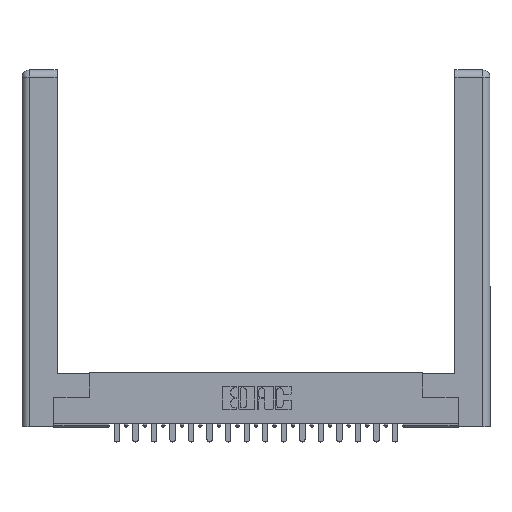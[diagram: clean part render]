
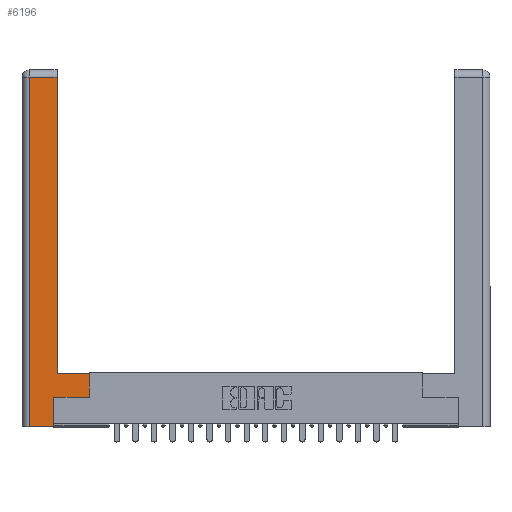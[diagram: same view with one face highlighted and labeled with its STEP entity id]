
A CAD part, top view. The second image highlights one B-rep face of the part: STEP entity #6196.
In plain terms, the highlighted planar face has unit normal (0, 0, 1).
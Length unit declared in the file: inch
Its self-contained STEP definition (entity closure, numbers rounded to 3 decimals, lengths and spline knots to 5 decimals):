
#140 = DIRECTION ( 'NONE',  ( 0., 1., 0. ) ) ;
#1581 = VERTEX_POINT ( 'NONE', #2366 ) ;
#2337 = DIRECTION ( 'NONE',  ( -1., 0., 0. ) ) ;
#2366 = CARTESIAN_POINT ( 'NONE',  ( 0.0615, 0., 0. ) ) ;
#3129 = ORIENTED_EDGE ( 'NONE', *, *, #21218, .T. ) ;
#3665 = FACE_OUTER_BOUND ( 'NONE', #14707, .T. ) ;
#3750 = CARTESIAN_POINT ( 'NONE',  ( 0.565, 0.245, 0. ) ) ;
#3934 = DIRECTION ( 'NONE',  ( 0., 1., 0. ) ) ;
#4056 = LINE ( 'NONE', #20084, #12375 ) ;
#4146 = EDGE_CURVE ( 'NONE', #20004, #16715, #7618, .T. ) ;
#4187 = PLANE ( 'NONE',  #8288 ) ;
#5728 = DIRECTION ( 'NONE',  ( -1., 0., 0. ) ) ;
#5800 = DIRECTION ( 'NONE',  ( 0., 0., -1. ) ) ;
#5822 = EDGE_CURVE ( 'NONE', #17576, #20868, #22886, .T. ) ;
#6196 = ADVANCED_FACE ( 'NONE', ( #3665 ), #4187, .F. ) ;
#6250 = DIRECTION ( 'NONE',  ( 0., -1., 0. ) ) ;
#6431 = CARTESIAN_POINT ( 'NONE',  ( 0.265, 0., 0. ) ) ;
#7618 = LINE ( 'NONE', #14719, #12907 ) ;
#7833 = VERTEX_POINT ( 'NONE', #8207 ) ;
#7955 = CARTESIAN_POINT ( 'NONE',  ( 0.0615, 0., 0. ) ) ;
#8207 = CARTESIAN_POINT ( 'NONE',  ( 0.265, 0.245, 0. ) ) ;
#8288 = AXIS2_PLACEMENT_3D ( 'NONE', #13018, #5800, #2337 ) ;
#8330 = DIRECTION ( 'NONE',  ( -1., 0., 0. ) ) ;
#8889 = ORIENTED_EDGE ( 'NONE', *, *, #21577, .T. ) ;
#9004 = VECTOR ( 'NONE', #18150, 39.37008 ) ;
#10523 = CARTESIAN_POINT ( 'NONE',  ( 0.265, 0.245, 0. ) ) ;
#11863 = EDGE_CURVE ( 'NONE', #13057, #7833, #12346, .T. ) ;
#12243 = CARTESIAN_POINT ( 'NONE',  ( 0.295, 0.45, 0. ) ) ;
#12346 = LINE ( 'NONE', #10523, #21276 ) ;
#12375 = VECTOR ( 'NONE', #3934, 39.37008 ) ;
#12907 = VECTOR ( 'NONE', #5728, 39.37008 ) ;
#13018 = CARTESIAN_POINT ( 'NONE',  ( 0., 0., 0. ) ) ;
#13057 = VERTEX_POINT ( 'NONE', #15611 ) ;
#14381 = VECTOR ( 'NONE', #19629, 39.37008 ) ;
#14426 = CARTESIAN_POINT ( 'NONE',  ( 0.295, 3., 0. ) ) ;
#14457 = ORIENTED_EDGE ( 'NONE', *, *, #16127, .T. ) ;
#14707 = EDGE_LOOP ( 'NONE', ( #19346, #19367, #3129, #15080, #16380, #8889, #14457, #16954 ) ) ;
#14719 = CARTESIAN_POINT ( 'NONE',  ( 0.0615, 2.94, 0. ) ) ;
#15080 = ORIENTED_EDGE ( 'NONE', *, *, #18209, .T. ) ;
#15426 = CARTESIAN_POINT ( 'NONE',  ( 0.565, 0.45, 0. ) ) ;
#15611 = CARTESIAN_POINT ( 'NONE',  ( 0.265, 0., 0. ) ) ;
#16127 = EDGE_CURVE ( 'NONE', #18651, #17576, #4056, .T. ) ;
#16380 = ORIENTED_EDGE ( 'NONE', *, *, #11863, .T. ) ;
#16715 = VERTEX_POINT ( 'NONE', #20460 ) ;
#16874 = LINE ( 'NONE', #17681, #14381 ) ;
#16954 = ORIENTED_EDGE ( 'NONE', *, *, #5822, .T. ) ;
#17320 = VECTOR ( 'NONE', #18893, 39.37008 ) ;
#17348 = EDGE_CURVE ( 'NONE', #20868, #20004, #20128, .T. ) ;
#17576 = VERTEX_POINT ( 'NONE', #15426 ) ;
#17681 = CARTESIAN_POINT ( 'NONE',  ( 0.565, 0.245, 0. ) ) ;
#18045 = CARTESIAN_POINT ( 'NONE',  ( 0.295, 2.94, 0. ) ) ;
#18150 = DIRECTION ( 'NONE',  ( 0., 1., 0. ) ) ;
#18209 = EDGE_CURVE ( 'NONE', #1581, #13057, #22062, .T. ) ;
#18651 = VERTEX_POINT ( 'NONE', #3750 ) ;
#18893 = DIRECTION ( 'NONE',  ( 1., 0., 0. ) ) ;
#19132 = CARTESIAN_POINT ( 'NONE',  ( 0.295, 0.45, 0. ) ) ;
#19346 = ORIENTED_EDGE ( 'NONE', *, *, #17348, .T. ) ;
#19367 = ORIENTED_EDGE ( 'NONE', *, *, #4146, .T. ) ;
#19629 = DIRECTION ( 'NONE',  ( 1., 0., 0. ) ) ;
#20004 = VERTEX_POINT ( 'NONE', #18045 ) ;
#20084 = CARTESIAN_POINT ( 'NONE',  ( 0.565, 0.45, 0. ) ) ;
#20128 = LINE ( 'NONE', #14426, #9004 ) ;
#20215 = LINE ( 'NONE', #7955, #22488 ) ;
#20460 = CARTESIAN_POINT ( 'NONE',  ( 0.0615, 2.94, 0. ) ) ;
#20868 = VERTEX_POINT ( 'NONE', #12243 ) ;
#20961 = VECTOR ( 'NONE', #8330, 39.37008 ) ;
#21218 = EDGE_CURVE ( 'NONE', #16715, #1581, #20215, .T. ) ;
#21276 = VECTOR ( 'NONE', #140, 39.37008 ) ;
#21577 = EDGE_CURVE ( 'NONE', #7833, #18651, #16874, .T. ) ;
#22062 = LINE ( 'NONE', #6431, #17320 ) ;
#22488 = VECTOR ( 'NONE', #6250, 39.37008 ) ;
#22886 = LINE ( 'NONE', #19132, #20961 ) ;
